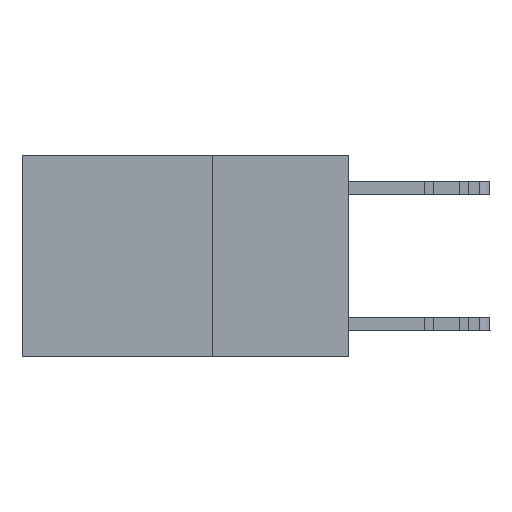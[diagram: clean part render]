
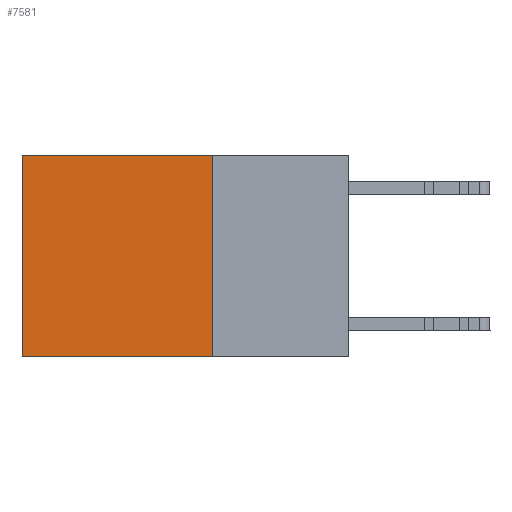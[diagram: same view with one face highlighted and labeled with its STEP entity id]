
A CAD part, left-side view. The second image highlights one B-rep face of the part: STEP entity #7581.
In plain terms, the highlighted planar face has unit normal (-1, 0, 0).
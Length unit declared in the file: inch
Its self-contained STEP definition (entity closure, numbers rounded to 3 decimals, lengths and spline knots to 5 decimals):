
#29 = DIRECTION ( 'NONE',  ( 0., 1., 0. ) ) ;
#459 = VECTOR ( 'NONE', #26956, 39.37008 ) ;
#1271 = VECTOR ( 'NONE', #22835, 39.37008 ) ;
#1706 = ORIENTED_EDGE ( 'NONE', *, *, #26684, .T. ) ;
#4980 = ORIENTED_EDGE ( 'NONE', *, *, #10447, .T. ) ;
#5310 = VERTEX_POINT ( 'NONE', #12381 ) ;
#5354 = EDGE_LOOP ( 'NONE', ( #1706, #14043, #23900, #4980 ) ) ;
#6106 = AXIS2_PLACEMENT_3D ( 'NONE', #6627, #21094, #9416 ) ;
#6627 = CARTESIAN_POINT ( 'NONE',  ( 0.2625, 0.25, 0. ) ) ;
#7316 = VECTOR ( 'NONE', #16790, 39.37008 ) ;
#7581 = ADVANCED_FACE ( 'NONE', ( #30019 ), #17925, .F. ) ;
#8351 = LINE ( 'NONE', #26865, #459 ) ;
#9416 = DIRECTION ( 'NONE',  ( 0., 0., -1. ) ) ;
#10063 = LINE ( 'NONE', #10978, #7316 ) ;
#10447 = EDGE_CURVE ( 'NONE', #5310, #23387, #16110, .T. ) ;
#10978 = CARTESIAN_POINT ( 'NONE',  ( 0.2625, 0.25, -0.37 ) ) ;
#11300 = CARTESIAN_POINT ( 'NONE',  ( 0.2625, 0.6, 0. ) ) ;
#11677 = CARTESIAN_POINT ( 'NONE',  ( 0.2625, 0.6, -0.37 ) ) ;
#11800 = CARTESIAN_POINT ( 'NONE',  ( 0.2625, 0.25, -0.37 ) ) ;
#11974 = EDGE_CURVE ( 'NONE', #27044, #14870, #10063, .T. ) ;
#12381 = CARTESIAN_POINT ( 'NONE',  ( 0.2625, 0.25, 0. ) ) ;
#13910 = VECTOR ( 'NONE', #29, 39.37008 ) ;
#14043 = ORIENTED_EDGE ( 'NONE', *, *, #11974, .F. ) ;
#14289 = EDGE_CURVE ( 'NONE', #5310, #27044, #28650, .T. ) ;
#14486 = CARTESIAN_POINT ( 'NONE',  ( 0.2625, 0.25, 0. ) ) ;
#14870 = VERTEX_POINT ( 'NONE', #11677 ) ;
#16110 = LINE ( 'NONE', #25202, #13910 ) ;
#16790 = DIRECTION ( 'NONE',  ( 0., 1., 0. ) ) ;
#17925 = PLANE ( 'NONE',  #6106 ) ;
#21094 = DIRECTION ( 'NONE',  ( 1., 0., 0. ) ) ;
#22835 = DIRECTION ( 'NONE',  ( 0., 0., -1. ) ) ;
#23387 = VERTEX_POINT ( 'NONE', #11300 ) ;
#23900 = ORIENTED_EDGE ( 'NONE', *, *, #14289, .F. ) ;
#25202 = CARTESIAN_POINT ( 'NONE',  ( 0.2625, 0.25, 0. ) ) ;
#26684 = EDGE_CURVE ( 'NONE', #23387, #14870, #8351, .T. ) ;
#26865 = CARTESIAN_POINT ( 'NONE',  ( 0.2625, 0.6, 0. ) ) ;
#26956 = DIRECTION ( 'NONE',  ( 0., 0., -1. ) ) ;
#27044 = VERTEX_POINT ( 'NONE', #11800 ) ;
#28650 = LINE ( 'NONE', #14486, #1271 ) ;
#30019 = FACE_OUTER_BOUND ( 'NONE', #5354, .T. ) ;
